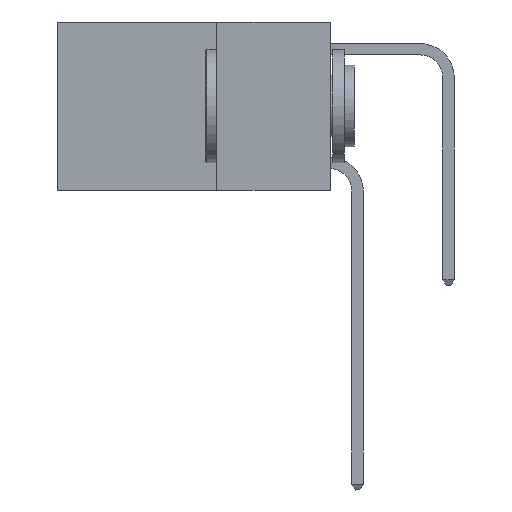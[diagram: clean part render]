
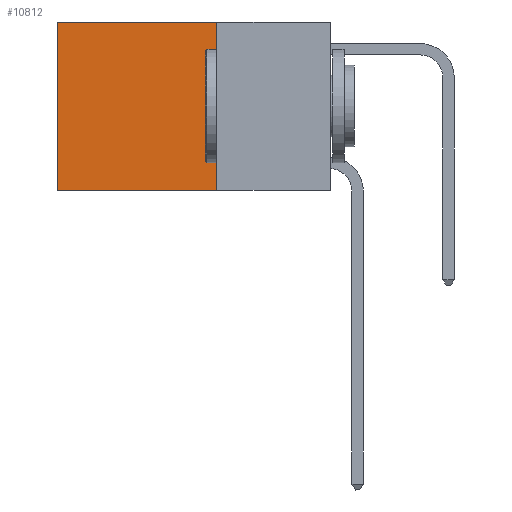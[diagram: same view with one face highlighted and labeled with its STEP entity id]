
A CAD part, left-side view. The second image highlights one B-rep face of the part: STEP entity #10812.
In plain terms, the highlighted planar face has unit normal (-1, 0, 0).
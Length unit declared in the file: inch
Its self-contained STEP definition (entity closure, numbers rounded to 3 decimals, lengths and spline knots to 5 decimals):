
#40 = LINE ( 'NONE', #9691, #5159 ) ;
#931 = PLANE ( 'NONE',  #9865 ) ;
#1213 = EDGE_CURVE ( 'NONE', #3907, #2070, #9553, .T. ) ;
#1537 = CARTESIAN_POINT ( 'NONE',  ( 0.2625, 0.6, 0. ) ) ;
#1582 = ORIENTED_EDGE ( 'NONE', *, *, #5520, .T. ) ;
#1755 = CARTESIAN_POINT ( 'NONE',  ( 0.2625, 0.25, -0.37 ) ) ;
#1820 = CARTESIAN_POINT ( 'NONE',  ( 0.2625, 0.6, -0.37 ) ) ;
#1829 = ORIENTED_EDGE ( 'NONE', *, *, #7228, .F. ) ;
#2070 = VERTEX_POINT ( 'NONE', #1537 ) ;
#2298 = CARTESIAN_POINT ( 'NONE',  ( 0.2625, 0.25, 0. ) ) ;
#2336 = LINE ( 'NONE', #5690, #4528 ) ;
#2502 = CARTESIAN_POINT ( 'NONE',  ( 0.2625, 0.25, 0. ) ) ;
#2827 = DIRECTION ( 'NONE',  ( 0., 1., 0. ) ) ;
#2940 = ORIENTED_EDGE ( 'NONE', *, *, #1213, .T. ) ;
#3490 = EDGE_LOOP ( 'NONE', ( #1582, #1829, #8091, #2940 ) ) ;
#3907 = VERTEX_POINT ( 'NONE', #2298 ) ;
#4528 = VECTOR ( 'NONE', #6684, 39.37008 ) ;
#4708 = DIRECTION ( 'NONE',  ( 0., 0., -1. ) ) ;
#4762 = CARTESIAN_POINT ( 'NONE',  ( 0.2625, 0.25, 0. ) ) ;
#5159 = VECTOR ( 'NONE', #10701, 39.37008 ) ;
#5202 = EDGE_CURVE ( 'NONE', #3907, #5287, #10898, .T. ) ;
#5287 = VERTEX_POINT ( 'NONE', #1755 ) ;
#5520 = EDGE_CURVE ( 'NONE', #2070, #8871, #40, .T. ) ;
#5690 = CARTESIAN_POINT ( 'NONE',  ( 0.2625, 0.25, -0.37 ) ) ;
#5702 = DIRECTION ( 'NONE',  ( 0., 0., -1. ) ) ;
#6684 = DIRECTION ( 'NONE',  ( 0., 1., 0. ) ) ;
#6918 = VECTOR ( 'NONE', #2827, 39.37008 ) ;
#7228 = EDGE_CURVE ( 'NONE', #5287, #8871, #2336, .T. ) ;
#8091 = ORIENTED_EDGE ( 'NONE', *, *, #5202, .F. ) ;
#8871 = VERTEX_POINT ( 'NONE', #1820 ) ;
#9553 = LINE ( 'NONE', #2502, #6918 ) ;
#9594 = CARTESIAN_POINT ( 'NONE',  ( 0.2625, 0.25, 0. ) ) ;
#9691 = CARTESIAN_POINT ( 'NONE',  ( 0.2625, 0.6, 0. ) ) ;
#9865 = AXIS2_PLACEMENT_3D ( 'NONE', #9594, #10608, #4708 ) ;
#10576 = VECTOR ( 'NONE', #5702, 39.37008 ) ;
#10608 = DIRECTION ( 'NONE',  ( 1., 0., 0. ) ) ;
#10701 = DIRECTION ( 'NONE',  ( 0., 0., -1. ) ) ;
#10812 = ADVANCED_FACE ( 'NONE', ( #12450 ), #931, .F. ) ;
#10898 = LINE ( 'NONE', #4762, #10576 ) ;
#12450 = FACE_OUTER_BOUND ( 'NONE', #3490, .T. ) ;
